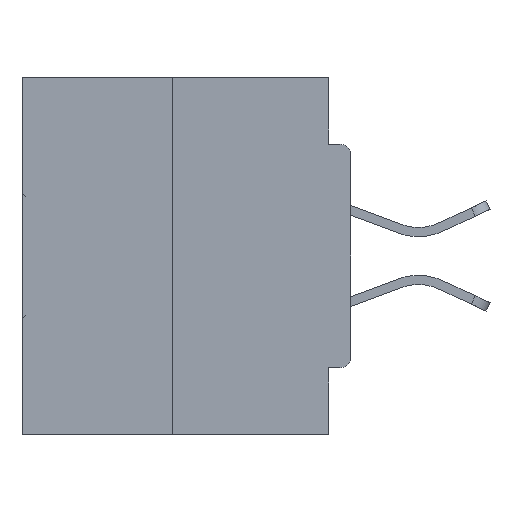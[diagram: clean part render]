
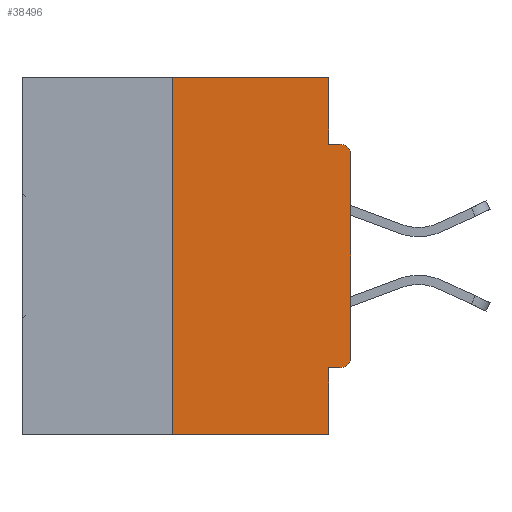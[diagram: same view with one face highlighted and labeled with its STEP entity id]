
A CAD part, left-side view. The second image highlights one B-rep face of the part: STEP entity #38496.
In plain terms, the highlighted planar face has unit normal (-1, 0, 0).
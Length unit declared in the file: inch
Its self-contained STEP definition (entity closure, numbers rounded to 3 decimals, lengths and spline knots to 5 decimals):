
#997 = VERTEX_POINT ( 'NONE', #35670 ) ;
#1735 = VERTEX_POINT ( 'NONE', #34111 ) ;
#2377 = ORIENTED_EDGE ( 'NONE', *, *, #5026, .F. ) ;
#3593 = EDGE_CURVE ( 'NONE', #1735, #997, #22440, .T. ) ;
#4127 = AXIS2_PLACEMENT_3D ( 'NONE', #6272, #6492, #19555 ) ;
#4457 = DIRECTION ( 'NONE',  ( -1., 0., 0. ) ) ;
#5026 = EDGE_CURVE ( 'NONE', #18826, #1735, #22349, .T. ) ;
#5059 = VERTEX_POINT ( 'NONE', #15947 ) ;
#5157 = ORIENTED_EDGE ( 'NONE', *, *, #23582, .F. ) ;
#6104 = DIRECTION ( 'NONE',  ( 0., 1., 0. ) ) ;
#6272 = CARTESIAN_POINT ( 'NONE',  ( 0., 0.46, 0. ) ) ;
#6334 = CARTESIAN_POINT ( 'NONE',  ( 0., 0., -0.0935 ) ) ;
#6456 = VECTOR ( 'NONE', #36369, 39.37008 ) ;
#6492 = DIRECTION ( 'NONE',  ( 1., 0., 0. ) ) ;
#7065 = CIRCLE ( 'NONE', #11851, 0.015 ) ;
#7266 = CARTESIAN_POINT ( 'NONE',  ( 0., 0.46, 0. ) ) ;
#7812 = DIRECTION ( 'NONE',  ( 0., 0., 1. ) ) ;
#8752 = EDGE_CURVE ( 'NONE', #28532, #41266, #33068, .T. ) ;
#8858 = EDGE_CURVE ( 'NONE', #41885, #28113, #20638, .T. ) ;
#10878 = ORIENTED_EDGE ( 'NONE', *, *, #8752, .F. ) ;
#11408 = LINE ( 'NONE', #24233, #24041 ) ;
#11851 = AXIS2_PLACEMENT_3D ( 'NONE', #26921, #4457, #17527 ) ;
#11874 = VECTOR ( 'NONE', #6104, 39.37008 ) ;
#12239 = CARTESIAN_POINT ( 'NONE',  ( 0., 0.031, 0. ) ) ;
#12692 = EDGE_CURVE ( 'NONE', #18826, #41885, #7065, .T. ) ;
#13578 = DIRECTION ( 'NONE',  ( 0., -1., 0. ) ) ;
#13710 = CARTESIAN_POINT ( 'NONE',  ( 0., 0.015, -0.1085 ) ) ;
#13713 = ORIENTED_EDGE ( 'NONE', *, *, #33856, .F. ) ;
#13809 = CARTESIAN_POINT ( 'NONE',  ( 0., 0., 0. ) ) ;
#15947 = CARTESIAN_POINT ( 'NONE',  ( 0., 0.25, 0. ) ) ;
#16815 = CIRCLE ( 'NONE', #17497, 0.015 ) ;
#17358 = VECTOR ( 'NONE', #24143, 39.37008 ) ;
#17497 = AXIS2_PLACEMENT_3D ( 'NONE', #13710, #23955, #33172 ) ;
#17527 = DIRECTION ( 'NONE',  ( 0., 0., -1. ) ) ;
#18103 = CARTESIAN_POINT ( 'NONE',  ( 0., 0.031, -0.0935 ) ) ;
#18207 = ORIENTED_EDGE ( 'NONE', *, *, #21350, .T. ) ;
#18826 = VERTEX_POINT ( 'NONE', #41279 ) ;
#18952 = EDGE_LOOP ( 'NONE', ( #20753, #13713, #18207, #35814, #2377, #21559, #41570, #30430, #10878, #5157 ) ) ;
#19555 = DIRECTION ( 'NONE',  ( 0., 0., -1. ) ) ;
#19767 = PLANE ( 'NONE',  #4127 ) ;
#20638 = LINE ( 'NONE', #13809, #22478 ) ;
#20731 = CARTESIAN_POINT ( 'NONE',  ( 0., 0.031, 0. ) ) ;
#20753 = ORIENTED_EDGE ( 'NONE', *, *, #25720, .F. ) ;
#20824 = CARTESIAN_POINT ( 'NONE',  ( 0., 0.25, -0.5 ) ) ;
#21350 = EDGE_CURVE ( 'NONE', #26669, #997, #26830, .T. ) ;
#21559 = ORIENTED_EDGE ( 'NONE', *, *, #12692, .T. ) ;
#22349 = LINE ( 'NONE', #32197, #11874 ) ;
#22440 = LINE ( 'NONE', #38724, #27878 ) ;
#22478 = VECTOR ( 'NONE', #7812, 39.37008 ) ;
#23226 = DIRECTION ( 'NONE',  ( 0., -1., 0. ) ) ;
#23305 = LINE ( 'NONE', #7266, #6456 ) ;
#23582 = EDGE_CURVE ( 'NONE', #41850, #28532, #36812, .T. ) ;
#23955 = DIRECTION ( 'NONE',  ( -1., 0., 0. ) ) ;
#24041 = VECTOR ( 'NONE', #28299, 39.37008 ) ;
#24143 = DIRECTION ( 'NONE',  ( 0., 0., -1. ) ) ;
#24233 = CARTESIAN_POINT ( 'NONE',  ( 0., 0.25, 0. ) ) ;
#24433 = CARTESIAN_POINT ( 'NONE',  ( 0., 0., -0.3915 ) ) ;
#25720 = EDGE_CURVE ( 'NONE', #5059, #41850, #23305, .T. ) ;
#26669 = VERTEX_POINT ( 'NONE', #20824 ) ;
#26830 = LINE ( 'NONE', #29832, #27030 ) ;
#26921 = CARTESIAN_POINT ( 'NONE',  ( 0., 0.015, -0.3915 ) ) ;
#27030 = VECTOR ( 'NONE', #13578, 39.37008 ) ;
#27878 = VECTOR ( 'NONE', #35299, 39.37008 ) ;
#28113 = VERTEX_POINT ( 'NONE', #37609 ) ;
#28299 = DIRECTION ( 'NONE',  ( 0., 0., 1. ) ) ;
#28532 = VERTEX_POINT ( 'NONE', #18103 ) ;
#29832 = CARTESIAN_POINT ( 'NONE',  ( 0., 0.46, -0.5 ) ) ;
#30246 = VECTOR ( 'NONE', #23226, 39.37008 ) ;
#30430 = ORIENTED_EDGE ( 'NONE', *, *, #31182, .T. ) ;
#31182 = EDGE_CURVE ( 'NONE', #28113, #41266, #16815, .T. ) ;
#32197 = CARTESIAN_POINT ( 'NONE',  ( 0., 0., -0.4065 ) ) ;
#33068 = LINE ( 'NONE', #6334, #30246 ) ;
#33172 = DIRECTION ( 'NONE',  ( 0., 0., -1. ) ) ;
#33856 = EDGE_CURVE ( 'NONE', #26669, #5059, #11408, .T. ) ;
#34111 = CARTESIAN_POINT ( 'NONE',  ( 0., 0.031, -0.4065 ) ) ;
#35299 = DIRECTION ( 'NONE',  ( 0., 0., -1. ) ) ;
#35670 = CARTESIAN_POINT ( 'NONE',  ( 0., 0.031, -0.5 ) ) ;
#35814 = ORIENTED_EDGE ( 'NONE', *, *, #3593, .F. ) ;
#36369 = DIRECTION ( 'NONE',  ( 0., -1., 0. ) ) ;
#36812 = LINE ( 'NONE', #20731, #17358 ) ;
#37609 = CARTESIAN_POINT ( 'NONE',  ( 0., 0., -0.1085 ) ) ;
#38496 = ADVANCED_FACE ( 'NONE', ( #39881 ), #19767, .F. ) ;
#38724 = CARTESIAN_POINT ( 'NONE',  ( 0., 0.031, -0.5 ) ) ;
#39881 = FACE_OUTER_BOUND ( 'NONE', #18952, .T. ) ;
#39940 = CARTESIAN_POINT ( 'NONE',  ( 0., 0.015, -0.0935 ) ) ;
#41266 = VERTEX_POINT ( 'NONE', #39940 ) ;
#41279 = CARTESIAN_POINT ( 'NONE',  ( 0., 0.015, -0.4065 ) ) ;
#41570 = ORIENTED_EDGE ( 'NONE', *, *, #8858, .T. ) ;
#41850 = VERTEX_POINT ( 'NONE', #12239 ) ;
#41885 = VERTEX_POINT ( 'NONE', #24433 ) ;
